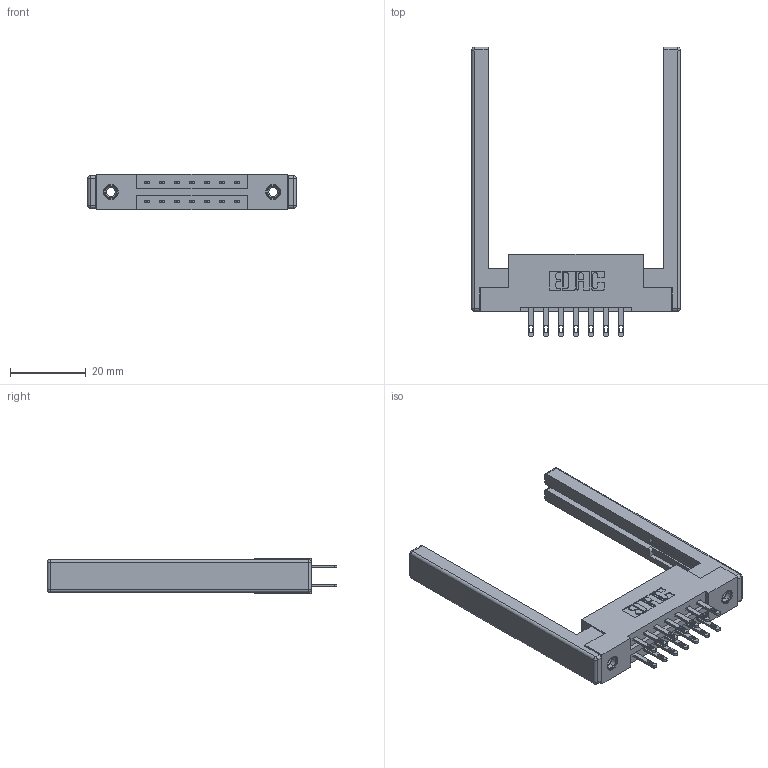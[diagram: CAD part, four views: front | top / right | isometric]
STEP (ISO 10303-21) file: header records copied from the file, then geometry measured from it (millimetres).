
FILE_DESCRIPTION (( 'STEP AP203' ), '1' );
FILE_NAME ('337-014-500-268.STEP', '2019-10-08T11:31:08', ( '' ), ( '' ), 'SwSTEP 2.0', 'SolidWorks 2016', '' );
FILE_SCHEMA (( 'CONFIG_CONTROL_DESIGN' ));
Length unit declared in the file: inch
Products named in the file (5): 345-250-001_345-250-001-102; 345-292-001_345-293-100; 337 Part_Flush Mounting Lugs - 0.156 Dia-TI; 307-220-068; 337-014-500-268
Assembly tree (19 placements, depth 2):
  337-014-500-268
    337 Part_Flush Mounting Lugs - 0.156 Dia-TI
    345-292-001_345-293-100  x14
    345-250-001_345-250-001-102  x2
    307-220-068  x2
Bounding box: 55.17 x 76.59 x 9.4 mm (x, y, z)
Volume: 9775.8 mm3; surface area: 9944.3 mm2
Topology: 19 solids, 19 shells, 968 faces, 2843 edges, 1874 vertices
Faces by surface type: plane 606, cylinder 338, cone 12, sphere 8, torus 4
Entity records: 12644 total; most frequent: CARTESIAN_POINT 2123, ORIENTED_EDGE 2048, DIRECTION 1942, EDGE_CURVE 1024, VECTOR 842, LINE 842, VERTEX_POINT 674, AXIS2_PLACEMENT_3D 550
